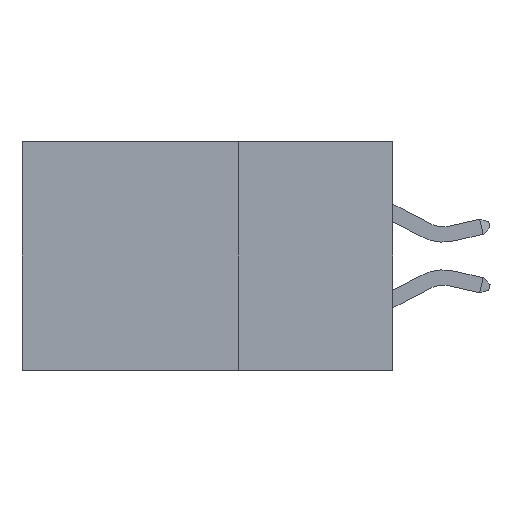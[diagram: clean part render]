
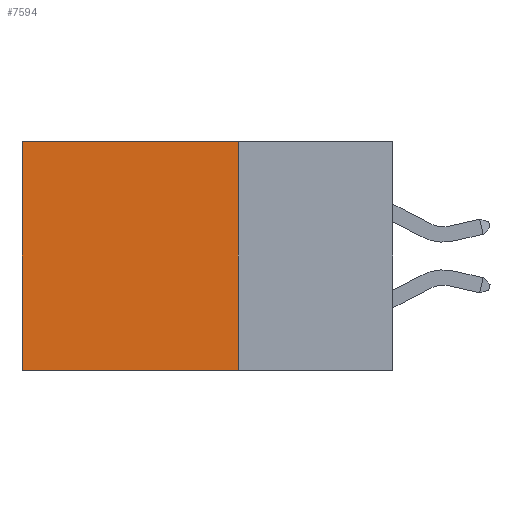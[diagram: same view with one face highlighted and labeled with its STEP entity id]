
A CAD part, left-side view. The second image highlights one B-rep face of the part: STEP entity #7594.
In plain terms, the highlighted planar face has unit normal (-1, 0, 0).
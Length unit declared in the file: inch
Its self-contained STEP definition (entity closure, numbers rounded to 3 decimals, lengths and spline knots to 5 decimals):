
#274 = CARTESIAN_POINT ( 'NONE',  ( 0.2875, 0.6, -0.37 ) ) ;
#369 = LINE ( 'NONE', #23891, #25658 ) ;
#2582 = DIRECTION ( 'NONE',  ( 0., 1., 0. ) ) ;
#2697 = EDGE_CURVE ( 'NONE', #28759, #27197, #24441, .T. ) ;
#6925 = CARTESIAN_POINT ( 'NONE',  ( 0.2875, 0.25, 0. ) ) ;
#7594 = ADVANCED_FACE ( 'NONE', ( #28894 ), #9149, .F. ) ;
#8675 = DIRECTION ( 'NONE',  ( 0., 1., 0. ) ) ;
#9149 = PLANE ( 'NONE',  #24479 ) ;
#9350 = VERTEX_POINT ( 'NONE', #23921 ) ;
#12334 = DIRECTION ( 'NONE',  ( 0., 0., -1. ) ) ;
#13299 = EDGE_CURVE ( 'NONE', #27197, #22771, #369, .T. ) ;
#14509 = ORIENTED_EDGE ( 'NONE', *, *, #2697, .T. ) ;
#14816 = EDGE_LOOP ( 'NONE', ( #18011, #26139, #25294, #14509 ) ) ;
#15024 = EDGE_CURVE ( 'NONE', #28759, #9350, #26673, .T. ) ;
#17829 = CARTESIAN_POINT ( 'NONE',  ( 0.2875, 0.6, 0. ) ) ;
#18011 = ORIENTED_EDGE ( 'NONE', *, *, #13299, .T. ) ;
#18118 = DIRECTION ( 'NONE',  ( 1., 0., 0. ) ) ;
#18620 = EDGE_CURVE ( 'NONE', #9350, #22771, #27553, .T. ) ;
#20094 = CARTESIAN_POINT ( 'NONE',  ( 0.2875, 0.25, 0. ) ) ;
#21001 = DIRECTION ( 'NONE',  ( 0., 0., -1. ) ) ;
#21364 = CARTESIAN_POINT ( 'NONE',  ( 0.2875, 0.25, -0.37 ) ) ;
#21566 = VECTOR ( 'NONE', #8675, 39.37008 ) ;
#21694 = CARTESIAN_POINT ( 'NONE',  ( 0.2875, 0.25, 0. ) ) ;
#22771 = VERTEX_POINT ( 'NONE', #274 ) ;
#23891 = CARTESIAN_POINT ( 'NONE',  ( 0.2875, 0.6, 0. ) ) ;
#23921 = CARTESIAN_POINT ( 'NONE',  ( 0.2875, 0.25, -0.37 ) ) ;
#24441 = LINE ( 'NONE', #20094, #21566 ) ;
#24479 = AXIS2_PLACEMENT_3D ( 'NONE', #6925, #18118, #21001 ) ;
#24981 = DIRECTION ( 'NONE',  ( 0., 0., -1. ) ) ;
#25082 = CARTESIAN_POINT ( 'NONE',  ( 0.2875, 0.25, 0. ) ) ;
#25294 = ORIENTED_EDGE ( 'NONE', *, *, #15024, .F. ) ;
#25658 = VECTOR ( 'NONE', #12334, 39.37008 ) ;
#26139 = ORIENTED_EDGE ( 'NONE', *, *, #18620, .F. ) ;
#26673 = LINE ( 'NONE', #25082, #28864 ) ;
#26795 = VECTOR ( 'NONE', #2582, 39.37008 ) ;
#27197 = VERTEX_POINT ( 'NONE', #17829 ) ;
#27553 = LINE ( 'NONE', #21364, #26795 ) ;
#28759 = VERTEX_POINT ( 'NONE', #21694 ) ;
#28864 = VECTOR ( 'NONE', #24981, 39.37008 ) ;
#28894 = FACE_OUTER_BOUND ( 'NONE', #14816, .T. ) ;
